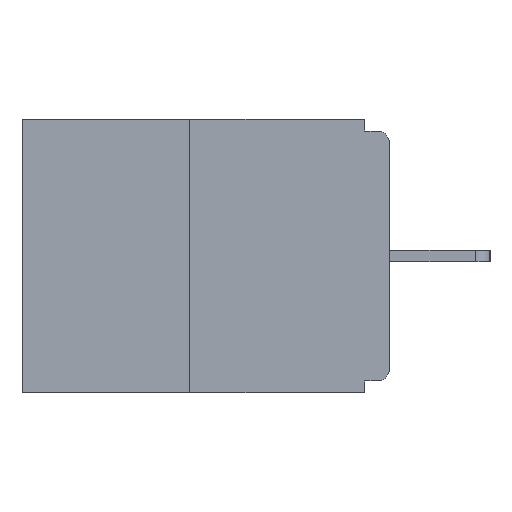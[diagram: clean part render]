
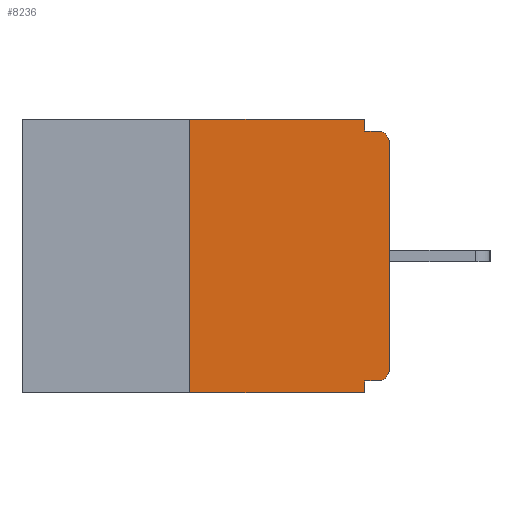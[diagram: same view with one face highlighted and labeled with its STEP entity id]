
A CAD part, left-side view. The second image highlights one B-rep face of the part: STEP entity #8236.
In plain terms, the highlighted planar face has unit normal (-1, 0, 0).
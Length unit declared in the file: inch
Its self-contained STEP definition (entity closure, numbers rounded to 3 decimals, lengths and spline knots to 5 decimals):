
#393 = DIRECTION ( 'NONE',  ( 0., -1., 0. ) ) ;
#911 = CARTESIAN_POINT ( 'NONE',  ( 0., 0.031, -0.343 ) ) ;
#932 = CARTESIAN_POINT ( 'NONE',  ( 0., 0.25, -0.343 ) ) ;
#1071 = CARTESIAN_POINT ( 'NONE',  ( 0., 0., -0.313 ) ) ;
#1422 = DIRECTION ( 'NONE',  ( -1., 0., 0. ) ) ;
#1448 = DIRECTION ( 'NONE',  ( 0., 1., 0. ) ) ;
#1490 = CARTESIAN_POINT ( 'NONE',  ( 0., 0., 0. ) ) ;
#1570 = VECTOR ( 'NONE', #393, 39.37008 ) ;
#1582 = VERTEX_POINT ( 'NONE', #10567 ) ;
#1613 = LINE ( 'NONE', #9933, #21029 ) ;
#1624 = DIRECTION ( 'NONE',  ( 0., 0., 1. ) ) ;
#2392 = CARTESIAN_POINT ( 'NONE',  ( 0., 0.031, -0.328 ) ) ;
#2832 = DIRECTION ( 'NONE',  ( 1., 0., 0. ) ) ;
#3064 = CARTESIAN_POINT ( 'NONE',  ( 0., 0., -0.328 ) ) ;
#3088 = DIRECTION ( 'NONE',  ( 0., 0., -1. ) ) ;
#3201 = VERTEX_POINT ( 'NONE', #2392 ) ;
#3294 = ORIENTED_EDGE ( 'NONE', *, *, #5437, .F. ) ;
#3633 = VERTEX_POINT ( 'NONE', #12313 ) ;
#3922 = ORIENTED_EDGE ( 'NONE', *, *, #13840, .F. ) ;
#4700 = EDGE_CURVE ( 'NONE', #19111, #14817, #8804, .T. ) ;
#5012 = DIRECTION ( 'NONE',  ( 0., 0., -1. ) ) ;
#5345 = CARTESIAN_POINT ( 'NONE',  ( 0., 0.25, 0. ) ) ;
#5349 = LINE ( 'NONE', #21785, #24262 ) ;
#5437 = EDGE_CURVE ( 'NONE', #19111, #22731, #7417, .T. ) ;
#5719 = AXIS2_PLACEMENT_3D ( 'NONE', #20178, #1422, #7968 ) ;
#6471 = DIRECTION ( 'NONE',  ( 0., -1., 0. ) ) ;
#6594 = EDGE_CURVE ( 'NONE', #3633, #8268, #9658, .T. ) ;
#7228 = PLANE ( 'NONE',  #21546 ) ;
#7417 = LINE ( 'NONE', #5345, #20561 ) ;
#7563 = EDGE_CURVE ( 'NONE', #3633, #3201, #24305, .T. ) ;
#7968 = DIRECTION ( 'NONE',  ( 0., 0., -1. ) ) ;
#8236 = ADVANCED_FACE ( 'NONE', ( #12956 ), #7228, .F. ) ;
#8268 = VERTEX_POINT ( 'NONE', #1071 ) ;
#8337 = AXIS2_PLACEMENT_3D ( 'NONE', #15679, #24580, #18025 ) ;
#8787 = VERTEX_POINT ( 'NONE', #23628 ) ;
#8804 = LINE ( 'NONE', #23199, #23858 ) ;
#9020 = CARTESIAN_POINT ( 'NONE',  ( 0., 0., -0.03 ) ) ;
#9516 = ORIENTED_EDGE ( 'NONE', *, *, #16752, .T. ) ;
#9587 = ORIENTED_EDGE ( 'NONE', *, *, #17441, .T. ) ;
#9658 = CIRCLE ( 'NONE', #5719, 0.015 ) ;
#9745 = CARTESIAN_POINT ( 'NONE',  ( 0., 0.25, 0. ) ) ;
#9933 = CARTESIAN_POINT ( 'NONE',  ( 0., 0.031, 0. ) ) ;
#10567 = CARTESIAN_POINT ( 'NONE',  ( 0., 0.031, 0. ) ) ;
#12171 = ORIENTED_EDGE ( 'NONE', *, *, #22397, .F. ) ;
#12313 = CARTESIAN_POINT ( 'NONE',  ( 0., 0.015, -0.328 ) ) ;
#12741 = VECTOR ( 'NONE', #1448, 39.37008 ) ;
#12956 = FACE_OUTER_BOUND ( 'NONE', #13099, .T. ) ;
#13099 = EDGE_LOOP ( 'NONE', ( #26250, #3294, #16373, #3922, #17642, #20300, #9587, #9516, #12171, #26435 ) ) ;
#13108 = LINE ( 'NONE', #25477, #1570 ) ;
#13366 = LINE ( 'NONE', #1490, #23697 ) ;
#13717 = DIRECTION ( 'NONE',  ( 0., -1., 0. ) ) ;
#13840 = EDGE_CURVE ( 'NONE', #3201, #14817, #26243, .T. ) ;
#14492 = VERTEX_POINT ( 'NONE', #21492 ) ;
#14817 = VERTEX_POINT ( 'NONE', #23096 ) ;
#15174 = EDGE_CURVE ( 'NONE', #1582, #8787, #1613, .T. ) ;
#15453 = CARTESIAN_POINT ( 'NONE',  ( 0., 0.46, 0. ) ) ;
#15663 = VERTEX_POINT ( 'NONE', #9020 ) ;
#15679 = CARTESIAN_POINT ( 'NONE',  ( 0., 0.015, -0.03 ) ) ;
#16373 = ORIENTED_EDGE ( 'NONE', *, *, #4700, .T. ) ;
#16752 = EDGE_CURVE ( 'NONE', #15663, #14492, #25403, .T. ) ;
#17058 = VECTOR ( 'NONE', #3088, 39.37008 ) ;
#17441 = EDGE_CURVE ( 'NONE', #8268, #15663, #13366, .T. ) ;
#17642 = ORIENTED_EDGE ( 'NONE', *, *, #7563, .F. ) ;
#18025 = DIRECTION ( 'NONE',  ( 0., 0., -1. ) ) ;
#19111 = VERTEX_POINT ( 'NONE', #932 ) ;
#20026 = DIRECTION ( 'NONE',  ( 0., 0., 1. ) ) ;
#20178 = CARTESIAN_POINT ( 'NONE',  ( 0., 0.015, -0.313 ) ) ;
#20300 = ORIENTED_EDGE ( 'NONE', *, *, #6594, .T. ) ;
#20561 = VECTOR ( 'NONE', #20026, 39.37008 ) ;
#21029 = VECTOR ( 'NONE', #21993, 39.37008 ) ;
#21492 = CARTESIAN_POINT ( 'NONE',  ( 0., 0.015, -0.015 ) ) ;
#21544 = EDGE_CURVE ( 'NONE', #22731, #1582, #13108, .T. ) ;
#21546 = AXIS2_PLACEMENT_3D ( 'NONE', #15453, #2832, #5012 ) ;
#21785 = CARTESIAN_POINT ( 'NONE',  ( 0., 0., -0.015 ) ) ;
#21993 = DIRECTION ( 'NONE',  ( 0., 0., -1. ) ) ;
#22397 = EDGE_CURVE ( 'NONE', #8787, #14492, #5349, .T. ) ;
#22731 = VERTEX_POINT ( 'NONE', #9745 ) ;
#23096 = CARTESIAN_POINT ( 'NONE',  ( 0., 0.031, -0.343 ) ) ;
#23199 = CARTESIAN_POINT ( 'NONE',  ( 0., 0.46, -0.343 ) ) ;
#23628 = CARTESIAN_POINT ( 'NONE',  ( 0., 0.031, -0.015 ) ) ;
#23697 = VECTOR ( 'NONE', #1624, 39.37008 ) ;
#23858 = VECTOR ( 'NONE', #6471, 39.37008 ) ;
#24262 = VECTOR ( 'NONE', #13717, 39.37008 ) ;
#24305 = LINE ( 'NONE', #3064, #12741 ) ;
#24580 = DIRECTION ( 'NONE',  ( -1., 0., 0. ) ) ;
#25403 = CIRCLE ( 'NONE', #8337, 0.015 ) ;
#25477 = CARTESIAN_POINT ( 'NONE',  ( 0., 0.46, 0. ) ) ;
#26243 = LINE ( 'NONE', #911, #17058 ) ;
#26250 = ORIENTED_EDGE ( 'NONE', *, *, #21544, .F. ) ;
#26435 = ORIENTED_EDGE ( 'NONE', *, *, #15174, .F. ) ;
